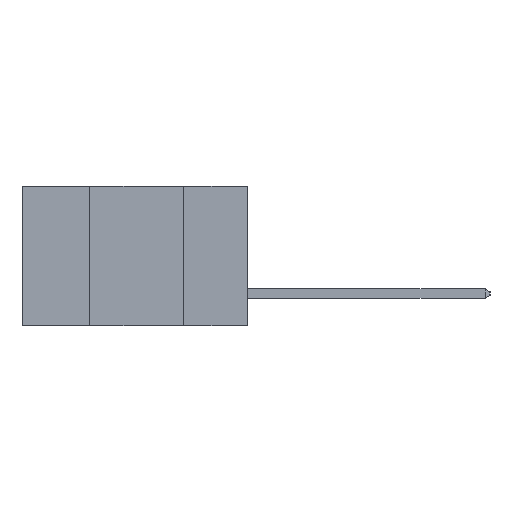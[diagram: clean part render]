
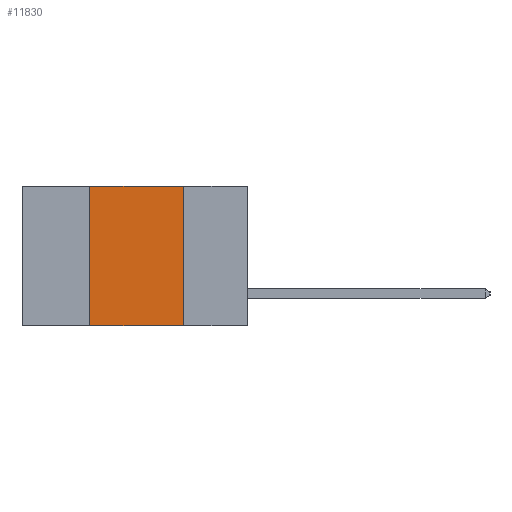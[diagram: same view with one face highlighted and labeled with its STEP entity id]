
A CAD part, left-side view. The second image highlights one B-rep face of the part: STEP entity #11830.
In plain terms, the highlighted planar face has unit normal (-1, 0, 0).
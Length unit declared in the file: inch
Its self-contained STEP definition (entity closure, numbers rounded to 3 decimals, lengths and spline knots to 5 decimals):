
#333 = EDGE_CURVE ( 'NONE', #20106, #20056, #6008, .T. ) ;
#1574 = EDGE_CURVE ( 'NONE', #23207, #7490, #18572, .T. ) ;
#1896 = VECTOR ( 'NONE', #17428, 39.37008 ) ;
#3003 = ORIENTED_EDGE ( 'NONE', *, *, #6025, .T. ) ;
#4348 = EDGE_CURVE ( 'NONE', #20056, #23207, #12317, .T. ) ;
#6008 = LINE ( 'NONE', #7205, #15044 ) ;
#6025 = EDGE_CURVE ( 'NONE', #20106, #7490, #24222, .T. ) ;
#6072 = CARTESIAN_POINT ( 'NONE',  ( 0., 0.17, -0.37 ) ) ;
#7205 = CARTESIAN_POINT ( 'NONE',  ( 0., 0.42, -0.37 ) ) ;
#7400 = PLANE ( 'NONE',  #18316 ) ;
#7490 = VERTEX_POINT ( 'NONE', #6072 ) ;
#7816 = DIRECTION ( 'NONE',  ( 0., 0., 1. ) ) ;
#9342 = DIRECTION ( 'NONE',  ( 1., 0., 0. ) ) ;
#11219 = CARTESIAN_POINT ( 'NONE',  ( 0., 0.6, 0. ) ) ;
#11830 = ADVANCED_FACE ( 'NONE', ( #19251 ), #7400, .F. ) ;
#12134 = EDGE_LOOP ( 'NONE', ( #24658, #13633, #24425, #3003 ) ) ;
#12317 = LINE ( 'NONE', #19052, #17423 ) ;
#13454 = VECTOR ( 'NONE', #18953, 39.37008 ) ;
#13633 = ORIENTED_EDGE ( 'NONE', *, *, #4348, .F. ) ;
#15044 = VECTOR ( 'NONE', #7816, 39.37008 ) ;
#15621 = CARTESIAN_POINT ( 'NONE',  ( 0., 0.42, 0. ) ) ;
#17093 = CARTESIAN_POINT ( 'NONE',  ( 0., 0.17, -0.37 ) ) ;
#17423 = VECTOR ( 'NONE', #18861, 39.37008 ) ;
#17428 = DIRECTION ( 'NONE',  ( 0., 0., -1. ) ) ;
#18316 = AXIS2_PLACEMENT_3D ( 'NONE', #11219, #9342, #22785 ) ;
#18572 = LINE ( 'NONE', #17093, #1896 ) ;
#18861 = DIRECTION ( 'NONE',  ( 0., -1., 0. ) ) ;
#18922 = CARTESIAN_POINT ( 'NONE',  ( 0., 0.6, -0.37 ) ) ;
#18953 = DIRECTION ( 'NONE',  ( 0., -1., 0. ) ) ;
#19052 = CARTESIAN_POINT ( 'NONE',  ( 0., 0.6, 0. ) ) ;
#19251 = FACE_OUTER_BOUND ( 'NONE', #12134, .T. ) ;
#19587 = CARTESIAN_POINT ( 'NONE',  ( 0., 0.42, -0.37 ) ) ;
#20056 = VERTEX_POINT ( 'NONE', #15621 ) ;
#20106 = VERTEX_POINT ( 'NONE', #19587 ) ;
#22537 = CARTESIAN_POINT ( 'NONE',  ( 0., 0.17, 0. ) ) ;
#22785 = DIRECTION ( 'NONE',  ( 0., 0., -1. ) ) ;
#23207 = VERTEX_POINT ( 'NONE', #22537 ) ;
#24222 = LINE ( 'NONE', #18922, #13454 ) ;
#24425 = ORIENTED_EDGE ( 'NONE', *, *, #333, .F. ) ;
#24658 = ORIENTED_EDGE ( 'NONE', *, *, #1574, .F. ) ;
